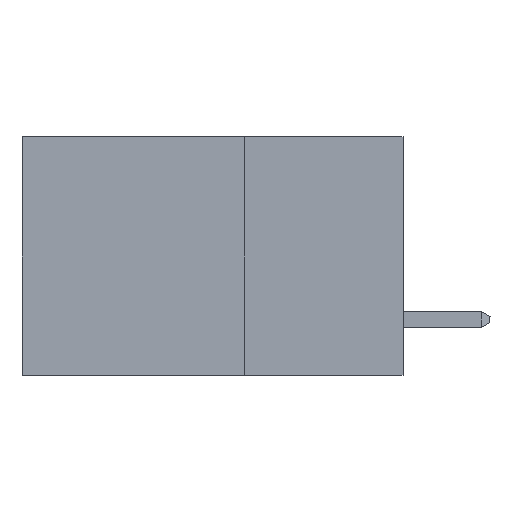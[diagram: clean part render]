
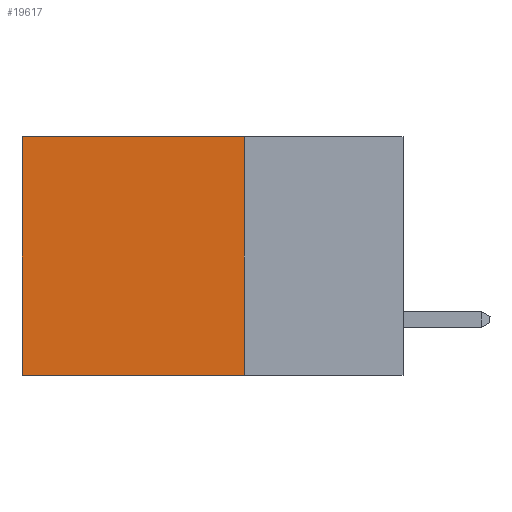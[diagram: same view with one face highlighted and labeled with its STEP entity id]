
A CAD part, left-side view. The second image highlights one B-rep face of the part: STEP entity #19617.
In plain terms, the highlighted planar face has unit normal (-1, 0, 0).
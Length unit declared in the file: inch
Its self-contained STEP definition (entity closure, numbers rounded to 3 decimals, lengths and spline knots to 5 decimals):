
#278 = LINE ( 'NONE', #12553, #3573 ) ;
#549 = VERTEX_POINT ( 'NONE', #7301 ) ;
#975 = PLANE ( 'NONE',  #16752 ) ;
#1339 = VECTOR ( 'NONE', #10679, 39.37008 ) ;
#2087 = VECTOR ( 'NONE', #20704, 39.37008 ) ;
#2622 = CARTESIAN_POINT ( 'NONE',  ( 0.2875, 0.6, -0.375 ) ) ;
#2930 = DIRECTION ( 'NONE',  ( 0., 0., -1. ) ) ;
#3009 = EDGE_CURVE ( 'NONE', #549, #12277, #16214, .T. ) ;
#3170 = LINE ( 'NONE', #5336, #3435 ) ;
#3435 = VECTOR ( 'NONE', #13274, 39.37008 ) ;
#3573 = VECTOR ( 'NONE', #2930, 39.37008 ) ;
#4569 = CARTESIAN_POINT ( 'NONE',  ( 0.2875, 0.25, -0.375 ) ) ;
#5336 = CARTESIAN_POINT ( 'NONE',  ( 0.2875, 0.25, 0. ) ) ;
#7301 = CARTESIAN_POINT ( 'NONE',  ( 0.2875, 0.6, 0. ) ) ;
#8132 = VERTEX_POINT ( 'NONE', #18142 ) ;
#8804 = EDGE_CURVE ( 'NONE', #8132, #549, #3170, .T. ) ;
#10679 = DIRECTION ( 'NONE',  ( 0., 0., -1. ) ) ;
#10701 = DIRECTION ( 'NONE',  ( 0., 0., -1. ) ) ;
#11245 = ORIENTED_EDGE ( 'NONE', *, *, #8804, .T. ) ;
#11574 = EDGE_LOOP ( 'NONE', ( #14519, #13095, #14473, #11245 ) ) ;
#12015 = EDGE_CURVE ( 'NONE', #8132, #14450, #278, .T. ) ;
#12213 = CARTESIAN_POINT ( 'NONE',  ( 0.2875, 0.25, -0.375 ) ) ;
#12277 = VERTEX_POINT ( 'NONE', #20597 ) ;
#12553 = CARTESIAN_POINT ( 'NONE',  ( 0.2875, 0.25, -0.375 ) ) ;
#13095 = ORIENTED_EDGE ( 'NONE', *, *, #18961, .F. ) ;
#13274 = DIRECTION ( 'NONE',  ( 0., 1., 0. ) ) ;
#14450 = VERTEX_POINT ( 'NONE', #18493 ) ;
#14473 = ORIENTED_EDGE ( 'NONE', *, *, #12015, .F. ) ;
#14519 = ORIENTED_EDGE ( 'NONE', *, *, #3009, .T. ) ;
#14883 = FACE_OUTER_BOUND ( 'NONE', #11574, .T. ) ;
#15454 = DIRECTION ( 'NONE',  ( 1., 0., 0. ) ) ;
#16214 = LINE ( 'NONE', #2622, #1339 ) ;
#16752 = AXIS2_PLACEMENT_3D ( 'NONE', #12213, #15454, #10701 ) ;
#18142 = CARTESIAN_POINT ( 'NONE',  ( 0.2875, 0.25, 0. ) ) ;
#18452 = LINE ( 'NONE', #4569, #2087 ) ;
#18493 = CARTESIAN_POINT ( 'NONE',  ( 0.2875, 0.25, -0.375 ) ) ;
#18961 = EDGE_CURVE ( 'NONE', #14450, #12277, #18452, .T. ) ;
#19617 = ADVANCED_FACE ( 'NONE', ( #14883 ), #975, .F. ) ;
#20597 = CARTESIAN_POINT ( 'NONE',  ( 0.2875, 0.6, -0.375 ) ) ;
#20704 = DIRECTION ( 'NONE',  ( 0., 1., 0. ) ) ;
